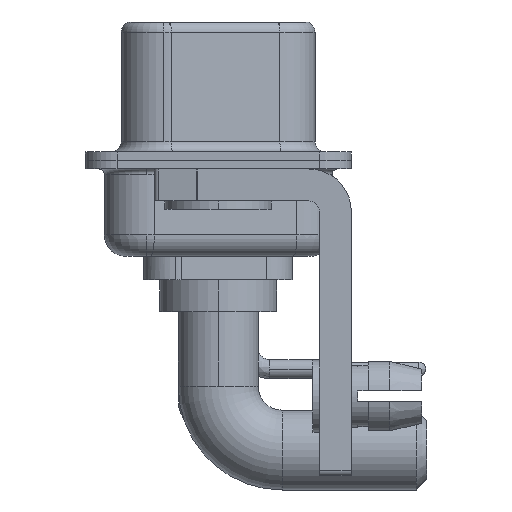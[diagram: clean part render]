
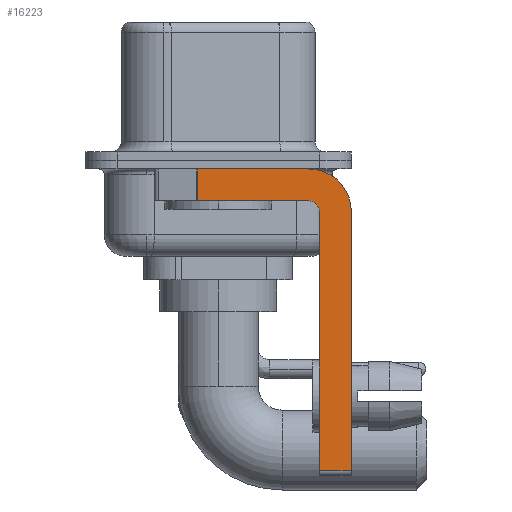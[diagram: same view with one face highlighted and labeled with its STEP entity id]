
A CAD part, left-side view. The second image highlights one B-rep face of the part: STEP entity #16223.
In plain terms, the highlighted planar face has unit normal (-1, 0, 0).
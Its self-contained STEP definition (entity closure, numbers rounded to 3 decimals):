
#228 = ORIENTED_EDGE ( 'NONE', *, *, #290, .F. ) ;
#290 = EDGE_CURVE ( 'NONE', #24601, #20689, #29380, .T. ) ;
#472 = VECTOR ( 'NONE', #2080, 1000. ) ;
#650 = CARTESIAN_POINT ( 'NONE',  ( -2.9, 0.978, -0.4 ) ) ;
#696 = LINE ( 'NONE', #26761, #10826 ) ;
#1579 = CARTESIAN_POINT ( 'NONE',  ( -2.9, -4.25, -1.9 ) ) ;
#1829 = DIRECTION ( 'NONE',  ( 0., 0., 1. ) ) ;
#2080 = DIRECTION ( 'NONE',  ( 0., 0., -1. ) ) ;
#2464 = DIRECTION ( 'NONE',  ( 0., 1., 0. ) ) ;
#3077 = CARTESIAN_POINT ( 'NONE',  ( -2.9, 0.978, -1.9 ) ) ;
#3745 = DIRECTION ( 'NONE',  ( 0., -1., 0. ) ) ;
#3750 = ORIENTED_EDGE ( 'NONE', *, *, #16068, .F. ) ;
#4749 = DIRECTION ( 'NONE',  ( 0., 0., -1. ) ) ;
#4864 = VECTOR ( 'NONE', #25846, 1000. ) ;
#5032 = VERTEX_POINT ( 'NONE', #11372 ) ;
#5770 = DIRECTION ( 'NONE',  ( 0., -1., 0. ) ) ;
#5835 = AXIS2_PLACEMENT_3D ( 'NONE', #9358, #18723, #4749 ) ;
#5841 = EDGE_CURVE ( 'NONE', #27484, #29142, #696, .T. ) ;
#6839 = CIRCLE ( 'NONE', #5835, 2. ) ;
#7889 = DIRECTION ( 'NONE',  ( 0., 0., -1. ) ) ;
#8163 = ORIENTED_EDGE ( 'NONE', *, *, #8206, .T. ) ;
#8206 = EDGE_CURVE ( 'NONE', #24600, #20689, #15252, .T. ) ;
#9308 = VERTEX_POINT ( 'NONE', #1579 ) ;
#9358 = CARTESIAN_POINT ( 'NONE',  ( -2.9, -4.25, -2.4 ) ) ;
#9739 = CARTESIAN_POINT ( 'NONE',  ( -2.9, -4.25, -2.4 ) ) ;
#9756 = EDGE_CURVE ( 'NONE', #24600, #5032, #24849, .T. ) ;
#10597 = DIRECTION ( 'NONE',  ( -1., 0., 0. ) ) ;
#10826 = VECTOR ( 'NONE', #5770, 1000. ) ;
#11372 = CARTESIAN_POINT ( 'NONE',  ( -2.9, -4.75, -2.4 ) ) ;
#11792 = EDGE_CURVE ( 'NONE', #29142, #24601, #6839, .T. ) ;
#11876 = DIRECTION ( 'NONE',  ( 1., 0., 0. ) ) ;
#11882 = CARTESIAN_POINT ( 'NONE',  ( -2.9, -6.25, -2.4 ) ) ;
#13040 = CARTESIAN_POINT ( 'NONE',  ( -2.9, -4.25, -2.4 ) ) ;
#13578 = LINE ( 'NONE', #22955, #472 ) ;
#13740 = VECTOR ( 'NONE', #2464, 1000. ) ;
#13882 = CARTESIAN_POINT ( 'NONE',  ( -2.9, -4.75, -14.55 ) ) ;
#14423 = CARTESIAN_POINT ( 'NONE',  ( -2.9, -4.25, -0.4 ) ) ;
#14480 = PLANE ( 'NONE',  #15393 ) ;
#15252 = LINE ( 'NONE', #27202, #16392 ) ;
#15393 = AXIS2_PLACEMENT_3D ( 'NONE', #9739, #11876, #7889 ) ;
#15966 = FACE_OUTER_BOUND ( 'NONE', #17949, .T. ) ;
#16068 = EDGE_CURVE ( 'NONE', #5032, #9308, #18824, .T. ) ;
#16193 = CARTESIAN_POINT ( 'NONE',  ( -2.9, -6.25, -2.4 ) ) ;
#16223 = ADVANCED_FACE ( 'NONE', ( #15966 ), #14480, .F. ) ;
#16392 = VECTOR ( 'NONE', #3745, 1000. ) ;
#17575 = ORIENTED_EDGE ( 'NONE', *, *, #5841, .F. ) ;
#17949 = EDGE_LOOP ( 'NONE', ( #17575, #18586, #20729, #3750, #20722, #8163, #228, #27456 ) ) ;
#18586 = ORIENTED_EDGE ( 'NONE', *, *, #24703, .T. ) ;
#18723 = DIRECTION ( 'NONE',  ( 1., 0., 0. ) ) ;
#18824 = CIRCLE ( 'NONE', #26636, 0.5 ) ;
#19183 = LINE ( 'NONE', #23495, #13740 ) ;
#19676 = DIRECTION ( 'NONE',  ( 0., 0., 1. ) ) ;
#20689 = VERTEX_POINT ( 'NONE', #22984 ) ;
#20722 = ORIENTED_EDGE ( 'NONE', *, *, #9756, .F. ) ;
#20729 = ORIENTED_EDGE ( 'NONE', *, *, #25713, .F. ) ;
#21099 = VECTOR ( 'NONE', #1829, 1000. ) ;
#22955 = CARTESIAN_POINT ( 'NONE',  ( -2.9, 0.978, -1.9 ) ) ;
#22984 = CARTESIAN_POINT ( 'NONE',  ( -2.9, -6.25, -14.55 ) ) ;
#23495 = CARTESIAN_POINT ( 'NONE',  ( -2.9, -4.25, -1.9 ) ) ;
#24600 = VERTEX_POINT ( 'NONE', #13882 ) ;
#24601 = VERTEX_POINT ( 'NONE', #16193 ) ;
#24703 = EDGE_CURVE ( 'NONE', #27484, #29264, #13578, .T. ) ;
#24849 = LINE ( 'NONE', #26977, #21099 ) ;
#25713 = EDGE_CURVE ( 'NONE', #9308, #29264, #19183, .T. ) ;
#25846 = DIRECTION ( 'NONE',  ( 0., 0., -1. ) ) ;
#26636 = AXIS2_PLACEMENT_3D ( 'NONE', #13040, #10597, #19676 ) ;
#26761 = CARTESIAN_POINT ( 'NONE',  ( -2.9, 3., -0.4 ) ) ;
#26977 = CARTESIAN_POINT ( 'NONE',  ( -2.9, -4.75, -14.8 ) ) ;
#27202 = CARTESIAN_POINT ( 'NONE',  ( -2.9, -4.25, -14.55 ) ) ;
#27456 = ORIENTED_EDGE ( 'NONE', *, *, #11792, .F. ) ;
#27484 = VERTEX_POINT ( 'NONE', #650 ) ;
#29142 = VERTEX_POINT ( 'NONE', #14423 ) ;
#29264 = VERTEX_POINT ( 'NONE', #3077 ) ;
#29380 = LINE ( 'NONE', #11882, #4864 ) ;
